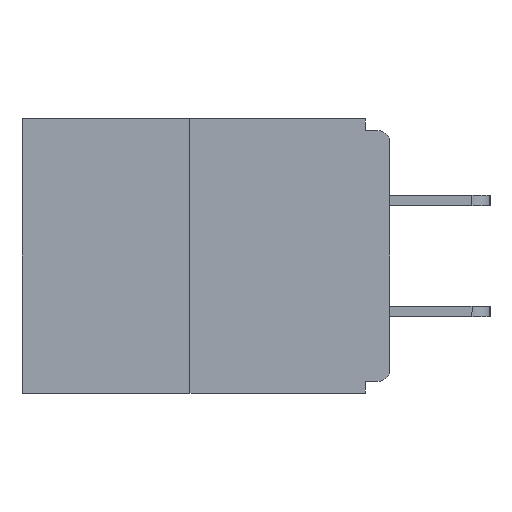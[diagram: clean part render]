
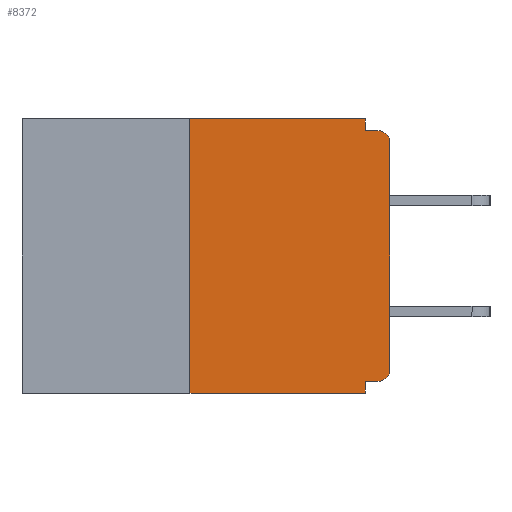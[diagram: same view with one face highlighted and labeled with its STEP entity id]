
A CAD part, left-side view. The second image highlights one B-rep face of the part: STEP entity #8372.
In plain terms, the highlighted planar face has unit normal (-1, 0, 0).
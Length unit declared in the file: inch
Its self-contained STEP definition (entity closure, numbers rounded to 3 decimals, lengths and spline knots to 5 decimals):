
#202 = CARTESIAN_POINT ( 'NONE',  ( 0., 0.015, -0.03 ) ) ;
#526 = DIRECTION ( 'NONE',  ( 1., 0., 0. ) ) ;
#756 = CARTESIAN_POINT ( 'NONE',  ( 0., 0.46, 0. ) ) ;
#1163 = VERTEX_POINT ( 'NONE', #12115 ) ;
#1512 = CARTESIAN_POINT ( 'NONE',  ( 0., 0.031, -0.015 ) ) ;
#1639 = VECTOR ( 'NONE', #10952, 39.37008 ) ;
#1912 = CARTESIAN_POINT ( 'NONE',  ( 0., 0.46, -0.343 ) ) ;
#1966 = VERTEX_POINT ( 'NONE', #11718 ) ;
#2156 = DIRECTION ( 'NONE',  ( 0., 0., -1. ) ) ;
#2412 = VECTOR ( 'NONE', #23256, 39.37008 ) ;
#2725 = AXIS2_PLACEMENT_3D ( 'NONE', #11938, #526, #13915 ) ;
#2899 = CARTESIAN_POINT ( 'NONE',  ( 0., 0.25, 0. ) ) ;
#2995 = LINE ( 'NONE', #6045, #2412 ) ;
#3043 = ORIENTED_EDGE ( 'NONE', *, *, #6806, .T. ) ;
#3067 = VERTEX_POINT ( 'NONE', #11915 ) ;
#3693 = EDGE_CURVE ( 'NONE', #3067, #22916, #20676, .T. ) ;
#3831 = DIRECTION ( 'NONE',  ( 0., -1., 0. ) ) ;
#4064 = VECTOR ( 'NONE', #23968, 39.37008 ) ;
#4247 = EDGE_LOOP ( 'NONE', ( #15836, #9626, #3043, #5698, #19928, #10315, #10429, #5305, #11303, #20564 ) ) ;
#4730 = VECTOR ( 'NONE', #3831, 39.37008 ) ;
#4811 = VERTEX_POINT ( 'NONE', #5961 ) ;
#5279 = EDGE_CURVE ( 'NONE', #23592, #1966, #13739, .T. ) ;
#5305 = ORIENTED_EDGE ( 'NONE', *, *, #13848, .T. ) ;
#5527 = DIRECTION ( 'NONE',  ( 0., 0., -1. ) ) ;
#5535 = EDGE_CURVE ( 'NONE', #4811, #3067, #16707, .T. ) ;
#5698 = ORIENTED_EDGE ( 'NONE', *, *, #3693, .F. ) ;
#5961 = CARTESIAN_POINT ( 'NONE',  ( 0., 0.015, -0.328 ) ) ;
#6045 = CARTESIAN_POINT ( 'NONE',  ( 0., 0.031, 0. ) ) ;
#6806 = EDGE_CURVE ( 'NONE', #23174, #22916, #8304, .T. ) ;
#7244 = VERTEX_POINT ( 'NONE', #8544 ) ;
#7303 = DIRECTION ( 'NONE',  ( 0., 1., 0. ) ) ;
#7863 = EDGE_CURVE ( 'NONE', #1163, #15300, #12767, .T. ) ;
#8304 = LINE ( 'NONE', #1912, #4730 ) ;
#8372 = ADVANCED_FACE ( 'NONE', ( #24040 ), #23048, .F. ) ;
#8537 = EDGE_CURVE ( 'NONE', #23174, #23592, #16269, .T. ) ;
#8544 = CARTESIAN_POINT ( 'NONE',  ( 0., 0.015, -0.015 ) ) ;
#9626 = ORIENTED_EDGE ( 'NONE', *, *, #8537, .F. ) ;
#10205 = EDGE_CURVE ( 'NONE', #12589, #7244, #12922, .T. ) ;
#10315 = ORIENTED_EDGE ( 'NONE', *, *, #11659, .T. ) ;
#10429 = ORIENTED_EDGE ( 'NONE', *, *, #7863, .T. ) ;
#10605 = CARTESIAN_POINT ( 'NONE',  ( 0., 0.031, -0.343 ) ) ;
#10952 = DIRECTION ( 'NONE',  ( 0., 0., -1. ) ) ;
#11303 = ORIENTED_EDGE ( 'NONE', *, *, #10205, .F. ) ;
#11659 = EDGE_CURVE ( 'NONE', #4811, #1163, #12239, .T. ) ;
#11718 = CARTESIAN_POINT ( 'NONE',  ( 0., 0.031, 0. ) ) ;
#11915 = CARTESIAN_POINT ( 'NONE',  ( 0., 0.031, -0.328 ) ) ;
#11938 = CARTESIAN_POINT ( 'NONE',  ( 0., 0.46, 0. ) ) ;
#12068 = AXIS2_PLACEMENT_3D ( 'NONE', #18741, #16924, #5527 ) ;
#12115 = CARTESIAN_POINT ( 'NONE',  ( 0., 0., -0.313 ) ) ;
#12239 = CIRCLE ( 'NONE', #12068, 0.015 ) ;
#12406 = CARTESIAN_POINT ( 'NONE',  ( 0., 0., -0.03 ) ) ;
#12589 = VERTEX_POINT ( 'NONE', #1512 ) ;
#12767 = LINE ( 'NONE', #23572, #17773 ) ;
#12922 = LINE ( 'NONE', #16303, #16780 ) ;
#13452 = VECTOR ( 'NONE', #7303, 39.37008 ) ;
#13498 = DIRECTION ( 'NONE',  ( -1., 0., 0. ) ) ;
#13739 = LINE ( 'NONE', #756, #23252 ) ;
#13848 = EDGE_CURVE ( 'NONE', #15300, #7244, #14833, .T. ) ;
#13915 = DIRECTION ( 'NONE',  ( 0., 0., -1. ) ) ;
#14833 = CIRCLE ( 'NONE', #19707, 0.015 ) ;
#14904 = CARTESIAN_POINT ( 'NONE',  ( 0., 0., -0.328 ) ) ;
#15300 = VERTEX_POINT ( 'NONE', #12406 ) ;
#15836 = ORIENTED_EDGE ( 'NONE', *, *, #5279, .F. ) ;
#16269 = LINE ( 'NONE', #2899, #4064 ) ;
#16303 = CARTESIAN_POINT ( 'NONE',  ( 0., 0., -0.015 ) ) ;
#16707 = LINE ( 'NONE', #14904, #13452 ) ;
#16780 = VECTOR ( 'NONE', #20011, 39.37008 ) ;
#16924 = DIRECTION ( 'NONE',  ( -1., 0., 0. ) ) ;
#17773 = VECTOR ( 'NONE', #21479, 39.37008 ) ;
#18741 = CARTESIAN_POINT ( 'NONE',  ( 0., 0.015, -0.313 ) ) ;
#19707 = AXIS2_PLACEMENT_3D ( 'NONE', #202, #13498, #2156 ) ;
#19826 = EDGE_CURVE ( 'NONE', #1966, #12589, #2995, .T. ) ;
#19870 = CARTESIAN_POINT ( 'NONE',  ( 0., 0.25, 0. ) ) ;
#19928 = ORIENTED_EDGE ( 'NONE', *, *, #5535, .F. ) ;
#20011 = DIRECTION ( 'NONE',  ( 0., -1., 0. ) ) ;
#20564 = ORIENTED_EDGE ( 'NONE', *, *, #19826, .F. ) ;
#20578 = CARTESIAN_POINT ( 'NONE',  ( 0., 0.25, -0.343 ) ) ;
#20676 = LINE ( 'NONE', #10605, #1639 ) ;
#21479 = DIRECTION ( 'NONE',  ( 0., 0., 1. ) ) ;
#21738 = CARTESIAN_POINT ( 'NONE',  ( 0., 0.031, -0.343 ) ) ;
#22916 = VERTEX_POINT ( 'NONE', #21738 ) ;
#23048 = PLANE ( 'NONE',  #2725 ) ;
#23174 = VERTEX_POINT ( 'NONE', #20578 ) ;
#23252 = VECTOR ( 'NONE', #23456, 39.37008 ) ;
#23256 = DIRECTION ( 'NONE',  ( 0., 0., -1. ) ) ;
#23456 = DIRECTION ( 'NONE',  ( 0., -1., 0. ) ) ;
#23572 = CARTESIAN_POINT ( 'NONE',  ( 0., 0., 0. ) ) ;
#23592 = VERTEX_POINT ( 'NONE', #19870 ) ;
#23968 = DIRECTION ( 'NONE',  ( 0., 0., 1. ) ) ;
#24040 = FACE_OUTER_BOUND ( 'NONE', #4247, .T. ) ;
